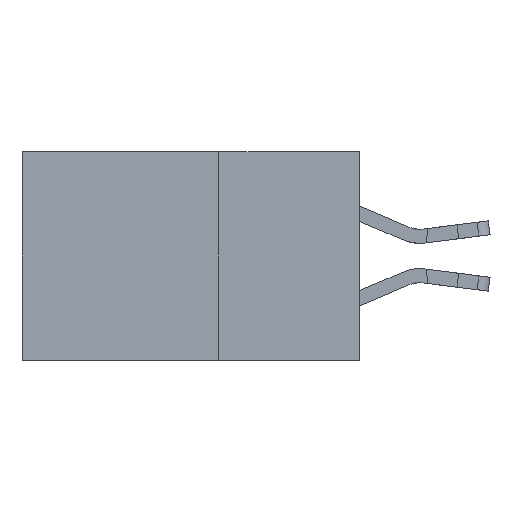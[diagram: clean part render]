
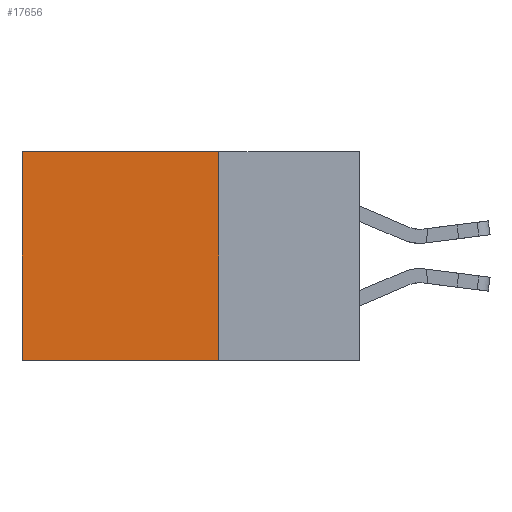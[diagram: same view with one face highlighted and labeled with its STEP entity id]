
A CAD part, left-side view. The second image highlights one B-rep face of the part: STEP entity #17656.
In plain terms, the highlighted planar face has unit normal (-1, 0, 0).
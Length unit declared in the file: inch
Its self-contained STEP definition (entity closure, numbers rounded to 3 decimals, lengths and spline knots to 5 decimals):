
#1723 = EDGE_LOOP ( 'NONE', ( #21261, #14005, #10559, #10673 ) ) ;
#4969 = CARTESIAN_POINT ( 'NONE',  ( 0.2875, 0.25, -0.37 ) ) ;
#5985 = CARTESIAN_POINT ( 'NONE',  ( 0.2875, 0.6, 0. ) ) ;
#6414 = VERTEX_POINT ( 'NONE', #5985 ) ;
#7538 = DIRECTION ( 'NONE',  ( 0., 0., -1. ) ) ;
#8002 = VERTEX_POINT ( 'NONE', #23051 ) ;
#10349 = DIRECTION ( 'NONE',  ( 0., 0., -1. ) ) ;
#10384 = DIRECTION ( 'NONE',  ( 0., 1., 0. ) ) ;
#10554 = EDGE_CURVE ( 'NONE', #25940, #15828, #20634, .T. ) ;
#10559 = ORIENTED_EDGE ( 'NONE', *, *, #10554, .F. ) ;
#10673 = ORIENTED_EDGE ( 'NONE', *, *, #19198, .T. ) ;
#10941 = DIRECTION ( 'NONE',  ( 0., 1., 0. ) ) ;
#10967 = DIRECTION ( 'NONE',  ( 0., 0., -1. ) ) ;
#11919 = VECTOR ( 'NONE', #7538, 39.37008 ) ;
#12798 = CARTESIAN_POINT ( 'NONE',  ( 0.2875, 0.6, 0. ) ) ;
#13512 = CARTESIAN_POINT ( 'NONE',  ( 0.2875, 0.25, 0. ) ) ;
#14005 = ORIENTED_EDGE ( 'NONE', *, *, #21254, .F. ) ;
#14419 = VECTOR ( 'NONE', #10967, 39.37008 ) ;
#15828 = VERTEX_POINT ( 'NONE', #31785 ) ;
#17656 = ADVANCED_FACE ( 'NONE', ( #22607 ), #23447, .F. ) ;
#18217 = CARTESIAN_POINT ( 'NONE',  ( 0.2875, 0.25, 0. ) ) ;
#18969 = LINE ( 'NONE', #12798, #11919 ) ;
#19198 = EDGE_CURVE ( 'NONE', #25940, #6414, #32414, .T. ) ;
#20634 = LINE ( 'NONE', #29394, #14419 ) ;
#21254 = EDGE_CURVE ( 'NONE', #15828, #8002, #21830, .T. ) ;
#21261 = ORIENTED_EDGE ( 'NONE', *, *, #27022, .T. ) ;
#21830 = LINE ( 'NONE', #4969, #29636 ) ;
#22607 = FACE_OUTER_BOUND ( 'NONE', #1723, .T. ) ;
#23051 = CARTESIAN_POINT ( 'NONE',  ( 0.2875, 0.6, -0.37 ) ) ;
#23447 = PLANE ( 'NONE',  #26384 ) ;
#23702 = VECTOR ( 'NONE', #10941, 39.37008 ) ;
#25940 = VERTEX_POINT ( 'NONE', #29297 ) ;
#26100 = DIRECTION ( 'NONE',  ( 1., 0., 0. ) ) ;
#26384 = AXIS2_PLACEMENT_3D ( 'NONE', #18217, #26100, #10349 ) ;
#27022 = EDGE_CURVE ( 'NONE', #6414, #8002, #18969, .T. ) ;
#29297 = CARTESIAN_POINT ( 'NONE',  ( 0.2875, 0.25, 0. ) ) ;
#29394 = CARTESIAN_POINT ( 'NONE',  ( 0.2875, 0.25, 0. ) ) ;
#29636 = VECTOR ( 'NONE', #10384, 39.37008 ) ;
#31785 = CARTESIAN_POINT ( 'NONE',  ( 0.2875, 0.25, -0.37 ) ) ;
#32414 = LINE ( 'NONE', #13512, #23702 ) ;
